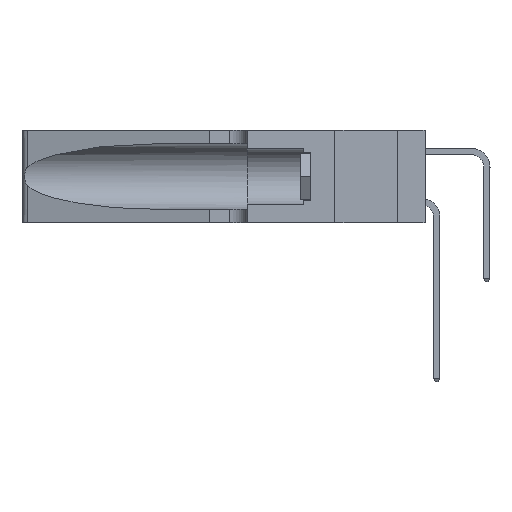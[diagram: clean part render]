
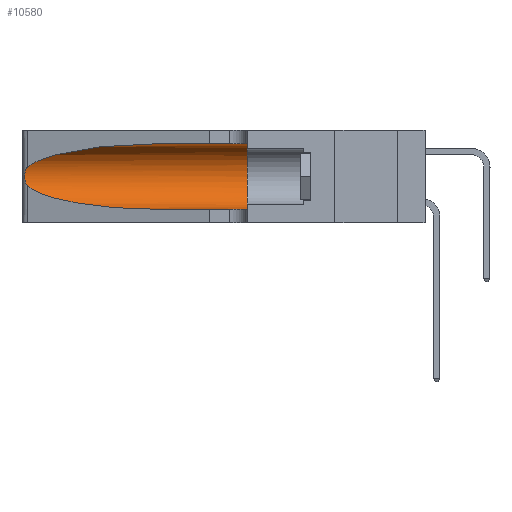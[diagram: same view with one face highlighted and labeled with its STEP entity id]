
A CAD part, left-side view. The second image highlights one B-rep face of the part: STEP entity #10580.
In plain terms, the highlighted cylindrical face has radius 3.308 mm (diameter 6.617 mm), a partial arc.
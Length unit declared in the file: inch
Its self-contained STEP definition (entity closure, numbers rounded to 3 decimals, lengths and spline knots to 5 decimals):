
#48 =( BOUNDED_CURVE ( )  B_SPLINE_CURVE ( 3, ( #13600, #25029, #15483, #3773 ),
 .UNSPECIFIED., .F., .F. ) 
 B_SPLINE_CURVE_WITH_KNOTS ( ( 4, 4 ),
 ( 1.5708, 2.84003 ),
 .UNSPECIFIED. ) 
 CURVE ( )  GEOMETRIC_REPRESENTATION_ITEM ( )  RATIONAL_B_SPLINE_CURVE ( ( 1., 0.87, 0.87, 1. ) ) 
 REPRESENTATION_ITEM ( '' )  );
#354 = CARTESIAN_POINT ( 'NONE',  ( 0.1305, 1.61858, 0.31525 ) ) ;
#1072 = CARTESIAN_POINT ( 'NONE',  ( 0.1305, 0.72297, 0.05475 ) ) ;
#1101 = CARTESIAN_POINT ( 'NONE',  ( 0.25787, 1.23484, 0.2124 ) ) ;
#1320 = EDGE_CURVE ( 'NONE', #17636, #13280, #8096, .T. ) ;
#1783 = DIRECTION ( 'NONE',  ( 0., -1., 0. ) ) ;
#2275 = B_SPLINE_CURVE_WITH_KNOTS ( 'NONE', 3,
 ( #14456, #23840, #8716, #1101, #2933, #13422, #16913, #21226, #23167, #7651, #19420, #3740, #13729, #5705 ),
 .UNSPECIFIED., .F., .F.,
 ( 4, 2, 2, 2, 2, 2, 4 ),
 ( 0., 0.00027, 0.00053, 0.00107, 0.0016, 0.00187, 0.00214 ),
 .UNSPECIFIED. ) ;
#2632 = VERTEX_POINT ( 'NONE', #5409 ) ;
#2933 = CARTESIAN_POINT ( 'NONE',  ( 0.25854, 1.2359, 0.20912 ) ) ;
#3408 = DIRECTION ( 'NONE',  ( 0., -1., 0. ) ) ;
#3562 = CIRCLE ( 'NONE', #19930, 0.13025 ) ;
#3740 = CARTESIAN_POINT ( 'NONE',  ( 0.25639, 1.23186, 0.15144 ) ) ;
#3773 = CARTESIAN_POINT ( 'NONE',  ( 0.25487, 1.22718, 0.22369 ) ) ;
#3844 = CARTESIAN_POINT ( 'NONE',  ( 0.1305, 1.61858, 0.185 ) ) ;
#4540 = DIRECTION ( 'NONE',  ( 0., 0., 1. ) ) ;
#4595 = VERTEX_POINT ( 'NONE', #13700 ) ;
#5106 = VERTEX_POINT ( 'NONE', #23123 ) ;
#5409 = CARTESIAN_POINT ( 'NONE',  ( 0.25487, 1.22718, 0.22369 ) ) ;
#5688 = ORIENTED_EDGE ( 'NONE', *, *, #16582, .T. ) ;
#5705 = CARTESIAN_POINT ( 'NONE',  ( 0.25487, 1.22718, 0.14631 ) ) ;
#5953 = FACE_OUTER_BOUND ( 'NONE', #15317, .T. ) ;
#6006 = CARTESIAN_POINT ( 'NONE',  ( 0.2373, 1.15595, 0.08982 ) ) ;
#6616 = DIRECTION ( 'NONE',  ( 0., -1., 0. ) ) ;
#7239 = ORIENTED_EDGE ( 'NONE', *, *, #14946, .F. ) ;
#7516 = DIRECTION ( 'NONE',  ( 0., 0., -1. ) ) ;
#7651 = CARTESIAN_POINT ( 'NONE',  ( 0.25856, 1.23593, 0.16098 ) ) ;
#8087 = EDGE_CURVE ( 'NONE', #2632, #17636, #2275, .T. ) ;
#8096 =( BOUNDED_CURVE ( )  B_SPLINE_CURVE ( 3, ( #12016, #6006, #16028, #21866 ),
 .UNSPECIFIED., .F., .F. ) 
 B_SPLINE_CURVE_WITH_KNOTS ( ( 4, 4 ),
 ( 3.44316, 4.71239 ),
 .UNSPECIFIED. ) 
 CURVE ( )  GEOMETRIC_REPRESENTATION_ITEM ( )  RATIONAL_B_SPLINE_CURVE ( ( 1., 0.87, 0.87, 1. ) ) 
 REPRESENTATION_ITEM ( '' )  );
#8716 = CARTESIAN_POINT ( 'NONE',  ( 0.25639, 1.23184, 0.21858 ) ) ;
#8766 = VECTOR ( 'NONE', #6616, 39.37008 ) ;
#9340 = CARTESIAN_POINT ( 'NONE',  ( 0.25487, 1.22718, 0.14631 ) ) ;
#10373 = ORIENTED_EDGE ( 'NONE', *, *, #8087, .T. ) ;
#10580 = ADVANCED_FACE ( 'NONE', ( #5953 ), #23044, .F. ) ;
#10932 = ORIENTED_EDGE ( 'NONE', *, *, #22436, .T. ) ;
#11148 = ORIENTED_EDGE ( 'NONE', *, *, #1320, .T. ) ;
#11201 = VERTEX_POINT ( 'NONE', #19401 ) ;
#12016 = CARTESIAN_POINT ( 'NONE',  ( 0.25487, 1.22718, 0.14631 ) ) ;
#13280 = VERTEX_POINT ( 'NONE', #1072 ) ;
#13422 = CARTESIAN_POINT ( 'NONE',  ( 0.26018, 1.23835, 0.19895 ) ) ;
#13600 = CARTESIAN_POINT ( 'NONE',  ( 0.1305, 0.72297, 0.31525 ) ) ;
#13700 = CARTESIAN_POINT ( 'NONE',  ( 0.1305, 0.35, 0.05475 ) ) ;
#13729 = CARTESIAN_POINT ( 'NONE',  ( 0.25555, 1.22993, 0.14849 ) ) ;
#13961 = LINE ( 'NONE', #22393, #8766 ) ;
#14456 = CARTESIAN_POINT ( 'NONE',  ( 0.25487, 1.22718, 0.22369 ) ) ;
#14946 = EDGE_CURVE ( 'NONE', #5106, #11201, #24374, .T. ) ;
#15317 = EDGE_LOOP ( 'NONE', ( #10932, #10373, #11148, #5688, #16781, #7239 ) ) ;
#15483 = CARTESIAN_POINT ( 'NONE',  ( 0.2373, 1.15595, 0.28018 ) ) ;
#16028 = CARTESIAN_POINT ( 'NONE',  ( 0.18966, 0.96281, 0.05475 ) ) ;
#16582 = EDGE_CURVE ( 'NONE', #13280, #4595, #13961, .T. ) ;
#16781 = ORIENTED_EDGE ( 'NONE', *, *, #17062, .F. ) ;
#16913 = CARTESIAN_POINT ( 'NONE',  ( 0.26075, 1.23896, 0.19203 ) ) ;
#17062 = EDGE_CURVE ( 'NONE', #11201, #4595, #3562, .T. ) ;
#17601 = AXIS2_PLACEMENT_3D ( 'NONE', #3844, #1783, #7516 ) ;
#17636 = VERTEX_POINT ( 'NONE', #9340 ) ;
#19401 = CARTESIAN_POINT ( 'NONE',  ( 0.1305, 0.35, 0.31525 ) ) ;
#19420 = CARTESIAN_POINT ( 'NONE',  ( 0.25789, 1.23486, 0.15765 ) ) ;
#19930 = AXIS2_PLACEMENT_3D ( 'NONE', #20068, #19979, #4540 ) ;
#19979 = DIRECTION ( 'NONE',  ( 0., 1., 0. ) ) ;
#20068 = CARTESIAN_POINT ( 'NONE',  ( 0.1305, 0.35, 0.185 ) ) ;
#20132 = VECTOR ( 'NONE', #3408, 39.37008 ) ;
#21226 = CARTESIAN_POINT ( 'NONE',  ( 0.26075, 1.23896, 0.178 ) ) ;
#21866 = CARTESIAN_POINT ( 'NONE',  ( 0.1305, 0.72297, 0.05475 ) ) ;
#22393 = CARTESIAN_POINT ( 'NONE',  ( 0.1305, 1.61858, 0.05475 ) ) ;
#22436 = EDGE_CURVE ( 'NONE', #5106, #2632, #48, .T. ) ;
#23044 = CYLINDRICAL_SURFACE ( 'NONE', #17601, 0.13025 ) ;
#23123 = CARTESIAN_POINT ( 'NONE',  ( 0.1305, 0.72297, 0.31525 ) ) ;
#23167 = CARTESIAN_POINT ( 'NONE',  ( 0.26017, 1.23833, 0.17102 ) ) ;
#23840 = CARTESIAN_POINT ( 'NONE',  ( 0.25555, 1.22994, 0.2215 ) ) ;
#24374 = LINE ( 'NONE', #354, #20132 ) ;
#25029 = CARTESIAN_POINT ( 'NONE',  ( 0.18966, 0.96281, 0.31525 ) ) ;
